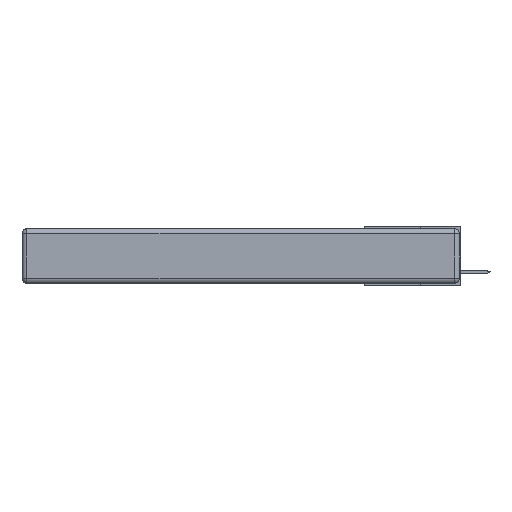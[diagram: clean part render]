
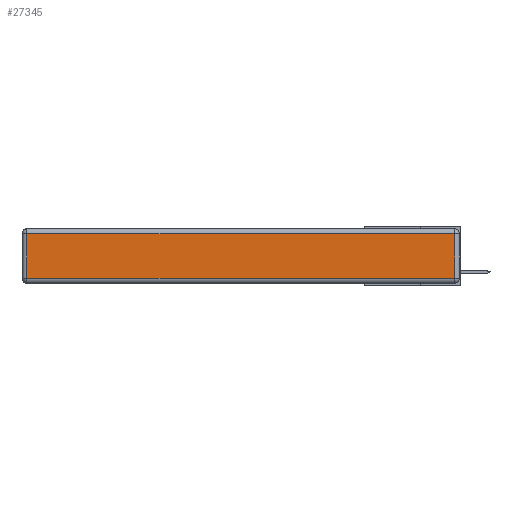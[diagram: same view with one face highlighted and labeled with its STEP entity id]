
A CAD part, left-side view. The second image highlights one B-rep face of the part: STEP entity #27345.
In plain terms, the highlighted planar face has unit normal (-1, 0, 0).
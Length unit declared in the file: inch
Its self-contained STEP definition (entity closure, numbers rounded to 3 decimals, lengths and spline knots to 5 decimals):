
#5367 = PLANE ( 'NONE',  #28276 ) ;
#5729 = DIRECTION ( 'NONE',  ( 0., 1., 0. ) ) ;
#6280 = EDGE_CURVE ( 'NONE', #24145, #6912, #17566, .T. ) ;
#6371 = LINE ( 'NONE', #23383, #33125 ) ;
#6912 = VERTEX_POINT ( 'NONE', #25646 ) ;
#7371 = VERTEX_POINT ( 'NONE', #8589 ) ;
#8146 = DIRECTION ( 'NONE',  ( 0., 0., -1. ) ) ;
#8589 = CARTESIAN_POINT ( 'NONE',  ( 0., 0.03, -0.313 ) ) ;
#10310 = DIRECTION ( 'NONE',  ( -1., 0., 0. ) ) ;
#10757 = DIRECTION ( 'NONE',  ( 0., 0., 1. ) ) ;
#12325 = EDGE_CURVE ( 'NONE', #7371, #24145, #15629, .T. ) ;
#13075 = LINE ( 'NONE', #14723, #18096 ) ;
#13364 = CARTESIAN_POINT ( 'NONE',  ( 0., 0., -0.343 ) ) ;
#14127 = ORIENTED_EDGE ( 'NONE', *, *, #12325, .T. ) ;
#14723 = CARTESIAN_POINT ( 'NONE',  ( 0., 0., -0.313 ) ) ;
#15629 = LINE ( 'NONE', #22319, #23587 ) ;
#17066 = CARTESIAN_POINT ( 'NONE',  ( 0., 0.03, -0.03 ) ) ;
#17548 = ORIENTED_EDGE ( 'NONE', *, *, #6280, .T. ) ;
#17566 = LINE ( 'NONE', #27013, #31810 ) ;
#17673 = FACE_OUTER_BOUND ( 'NONE', #20383, .T. ) ;
#18096 = VECTOR ( 'NONE', #28373, 39.37008 ) ;
#19981 = ORIENTED_EDGE ( 'NONE', *, *, #31397, .T. ) ;
#20233 = ORIENTED_EDGE ( 'NONE', *, *, #27539, .T. ) ;
#20383 = EDGE_LOOP ( 'NONE', ( #20233, #14127, #17548, #19981 ) ) ;
#22319 = CARTESIAN_POINT ( 'NONE',  ( 0., 0.03, -0.343 ) ) ;
#22560 = DIRECTION ( 'NONE',  ( 0., 0., 1. ) ) ;
#23383 = CARTESIAN_POINT ( 'NONE',  ( 0., 2.72, -0.343 ) ) ;
#23587 = VECTOR ( 'NONE', #22560, 39.37008 ) ;
#24145 = VERTEX_POINT ( 'NONE', #17066 ) ;
#25646 = CARTESIAN_POINT ( 'NONE',  ( 0., 2.72, -0.03 ) ) ;
#27013 = CARTESIAN_POINT ( 'NONE',  ( 0., 2.75, -0.03 ) ) ;
#27345 = ADVANCED_FACE ( 'NONE', ( #17673 ), #5367, .T. ) ;
#27539 = EDGE_CURVE ( 'NONE', #29806, #7371, #13075, .T. ) ;
#28276 = AXIS2_PLACEMENT_3D ( 'NONE', #13364, #10310, #10757 ) ;
#28373 = DIRECTION ( 'NONE',  ( 0., -1., 0. ) ) ;
#29806 = VERTEX_POINT ( 'NONE', #32754 ) ;
#31397 = EDGE_CURVE ( 'NONE', #6912, #29806, #6371, .T. ) ;
#31810 = VECTOR ( 'NONE', #5729, 39.37008 ) ;
#32754 = CARTESIAN_POINT ( 'NONE',  ( 0., 2.72, -0.313 ) ) ;
#33125 = VECTOR ( 'NONE', #8146, 39.37008 ) ;
